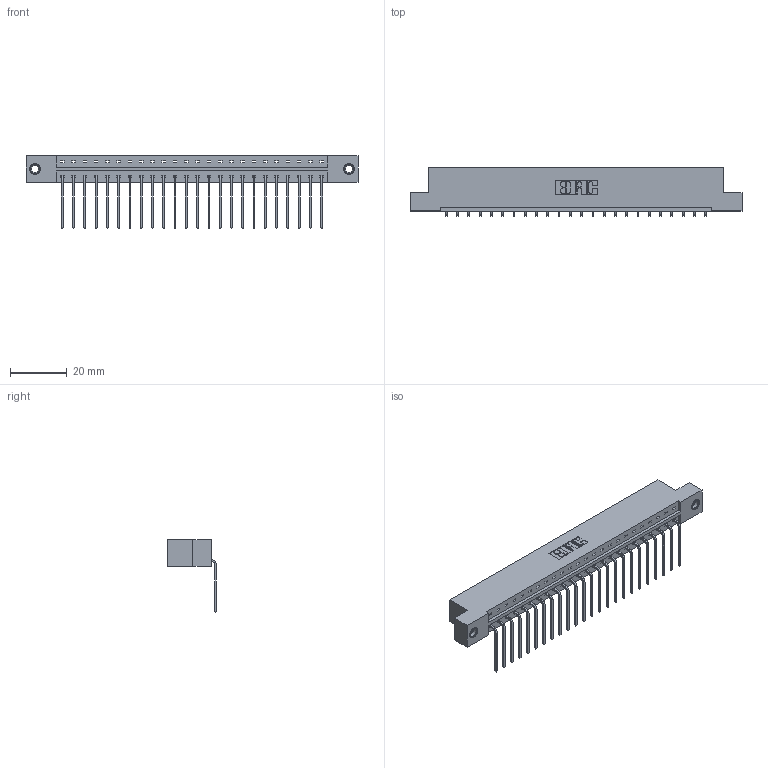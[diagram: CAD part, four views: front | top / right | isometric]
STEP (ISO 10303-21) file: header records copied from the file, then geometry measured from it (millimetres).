
FILE_DESCRIPTION (( 'STEP AP203' ), '1' );
FILE_NAME ('833-024-559-107.STEP', '2020-06-01T22:37:42', ( '' ), ( '' ), 'SwSTEP 2.0', 'SolidWorks 2020', '' );
FILE_SCHEMA (( 'CONFIG_CONTROL_DESIGN' ));
Length unit declared in the file: inch
Products named in the file (4): 833-024-559-107; 345-292-001_558 559 Tail - 1; 833 Part_Flush - .156 Dia - TI; 345-250-001_345-250-005-103
Assembly tree (27 placements, depth 2):
  833-024-559-107
    833 Part_Flush - .156 Dia - TI
    345-292-001_558 559 Tail - 1  x24
    345-250-001_345-250-005-103  x2
Bounding box: 116.64 x 17.09 x 25.53 mm (x, y, z)
Volume: 11648.6 mm3; surface area: 13013.6 mm2
Topology: 27 solids, 27 shells, 1614 faces, 4815 edges, 3170 vertices
Faces by surface type: plane 1158, cylinder 440, cone 12, torus 4
Entity records: 18270 total; most frequent: CARTESIAN_POINT 3137, ORIENTED_EDGE 3090, DIRECTION 2715, EDGE_CURVE 1545, LINE 1397, VECTOR 1397, VERTEX_POINT 1024, AXIS2_PLACEMENT_3D 659
